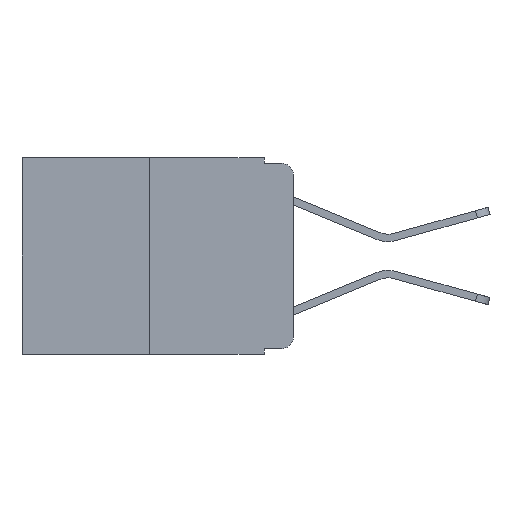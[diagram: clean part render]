
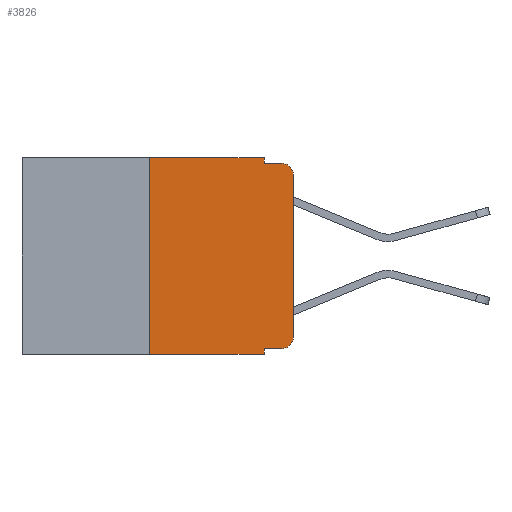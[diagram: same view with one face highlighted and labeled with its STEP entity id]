
A CAD part, left-side view. The second image highlights one B-rep face of the part: STEP entity #3826.
In plain terms, the highlighted planar face has unit normal (-1, 0, 0).
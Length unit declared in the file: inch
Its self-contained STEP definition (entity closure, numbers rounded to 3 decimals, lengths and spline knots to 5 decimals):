
#306 = CIRCLE ( 'NONE', #18237, 0.02 ) ;
#406 = VERTEX_POINT ( 'NONE', #5107 ) ;
#721 = DIRECTION ( 'NONE',  ( 0., -1., 0. ) ) ;
#767 = DIRECTION ( 'NONE',  ( 0., 0., -1. ) ) ;
#1211 = DIRECTION ( 'NONE',  ( 0., -1., 0. ) ) ;
#1782 = DIRECTION ( 'NONE',  ( 0., 0., -1. ) ) ;
#2209 = VERTEX_POINT ( 'NONE', #18327 ) ;
#2670 = VECTOR ( 'NONE', #22413, 39.37008 ) ;
#2703 = DIRECTION ( 'NONE',  ( -1., 0., 0. ) ) ;
#2939 = VECTOR ( 'NONE', #13207, 39.37008 ) ;
#3007 = CARTESIAN_POINT ( 'NONE',  ( 0., 0., 0. ) ) ;
#3672 = LINE ( 'NONE', #7604, #4236 ) ;
#3826 = ADVANCED_FACE ( 'NONE', ( #13907 ), #5703, .F. ) ;
#4138 = CARTESIAN_POINT ( 'NONE',  ( 0., 0.25, 0. ) ) ;
#4236 = VECTOR ( 'NONE', #19993, 39.37008 ) ;
#4844 = ORIENTED_EDGE ( 'NONE', *, *, #16726, .F. ) ;
#4916 = EDGE_CURVE ( 'NONE', #406, #8675, #20185, .T. ) ;
#4988 = VECTOR ( 'NONE', #721, 39.37008 ) ;
#5107 = CARTESIAN_POINT ( 'NONE',  ( 0., 0.25, -0.343 ) ) ;
#5152 = VECTOR ( 'NONE', #1782, 39.37008 ) ;
#5670 = ORIENTED_EDGE ( 'NONE', *, *, #21450, .F. ) ;
#5703 = PLANE ( 'NONE',  #8848 ) ;
#6111 = VECTOR ( 'NONE', #10324, 39.37008 ) ;
#6746 = EDGE_CURVE ( 'NONE', #7507, #6897, #306, .T. ) ;
#6845 = ORIENTED_EDGE ( 'NONE', *, *, #15632, .F. ) ;
#6897 = VERTEX_POINT ( 'NONE', #14021 ) ;
#7507 = VERTEX_POINT ( 'NONE', #19129 ) ;
#7604 = CARTESIAN_POINT ( 'NONE',  ( 0., 0.051, -0.01 ) ) ;
#7939 = EDGE_CURVE ( 'NONE', #21183, #7507, #10898, .T. ) ;
#7943 = CARTESIAN_POINT ( 'NONE',  ( 0., 0.051, -0.333 ) ) ;
#8013 = CARTESIAN_POINT ( 'NONE',  ( 0., 0.473, 0. ) ) ;
#8180 = DIRECTION ( 'NONE',  ( 0., 0., -1. ) ) ;
#8362 = LINE ( 'NONE', #9978, #13095 ) ;
#8675 = VERTEX_POINT ( 'NONE', #19466 ) ;
#8848 = AXIS2_PLACEMENT_3D ( 'NONE', #8013, #17214, #8180 ) ;
#9668 = ORIENTED_EDGE ( 'NONE', *, *, #15588, .T. ) ;
#9942 = ORIENTED_EDGE ( 'NONE', *, *, #7939, .T. ) ;
#9978 = CARTESIAN_POINT ( 'NONE',  ( 0., 0.051, 0. ) ) ;
#10151 = CARTESIAN_POINT ( 'NONE',  ( 0., 0., -0.313 ) ) ;
#10163 = VERTEX_POINT ( 'NONE', #11157 ) ;
#10324 = DIRECTION ( 'NONE',  ( 0., 0., 1. ) ) ;
#10366 = CARTESIAN_POINT ( 'NONE',  ( 0., 0.473, -0.343 ) ) ;
#10557 = LINE ( 'NONE', #10953, #5152 ) ;
#10720 = CIRCLE ( 'NONE', #17470, 0.02 ) ;
#10737 = CARTESIAN_POINT ( 'NONE',  ( 0., 0.02, -0.333 ) ) ;
#10898 = LINE ( 'NONE', #3007, #6111 ) ;
#10953 = CARTESIAN_POINT ( 'NONE',  ( 0., 0.051, 0. ) ) ;
#11157 = CARTESIAN_POINT ( 'NONE',  ( 0., 0.051, -0.01 ) ) ;
#11743 = DIRECTION ( 'NONE',  ( -1., 0., 0. ) ) ;
#11892 = CARTESIAN_POINT ( 'NONE',  ( 0., 0.25, 0. ) ) ;
#13095 = VECTOR ( 'NONE', #20552, 39.37008 ) ;
#13207 = DIRECTION ( 'NONE',  ( 0., 0., 1. ) ) ;
#13486 = CARTESIAN_POINT ( 'NONE',  ( 0., 0.051, -0.333 ) ) ;
#13560 = CARTESIAN_POINT ( 'NONE',  ( 0., 0.02, -0.03 ) ) ;
#13700 = LINE ( 'NONE', #4138, #2939 ) ;
#13907 = FACE_OUTER_BOUND ( 'NONE', #20303, .T. ) ;
#14021 = CARTESIAN_POINT ( 'NONE',  ( 0., 0.02, -0.01 ) ) ;
#14376 = EDGE_CURVE ( 'NONE', #21961, #21183, #10720, .T. ) ;
#14422 = VERTEX_POINT ( 'NONE', #11892 ) ;
#14671 = ORIENTED_EDGE ( 'NONE', *, *, #6746, .T. ) ;
#15352 = DIRECTION ( 'NONE',  ( 0., 0., -1. ) ) ;
#15588 = EDGE_CURVE ( 'NONE', #22804, #21961, #18105, .T. ) ;
#15632 = EDGE_CURVE ( 'NONE', #14422, #2209, #17564, .T. ) ;
#16633 = VECTOR ( 'NONE', #1211, 39.37008 ) ;
#16726 = EDGE_CURVE ( 'NONE', #22804, #8675, #8362, .T. ) ;
#17214 = DIRECTION ( 'NONE',  ( 1., 0., 0. ) ) ;
#17470 = AXIS2_PLACEMENT_3D ( 'NONE', #22300, #11743, #767 ) ;
#17564 = LINE ( 'NONE', #22333, #2670 ) ;
#17962 = ORIENTED_EDGE ( 'NONE', *, *, #4916, .T. ) ;
#18105 = LINE ( 'NONE', #13486, #4988 ) ;
#18237 = AXIS2_PLACEMENT_3D ( 'NONE', #13560, #2703, #15352 ) ;
#18327 = CARTESIAN_POINT ( 'NONE',  ( 0., 0.051, 0. ) ) ;
#19074 = ORIENTED_EDGE ( 'NONE', *, *, #14376, .T. ) ;
#19086 = EDGE_CURVE ( 'NONE', #406, #14422, #13700, .T. ) ;
#19129 = CARTESIAN_POINT ( 'NONE',  ( 0., 0., -0.03 ) ) ;
#19466 = CARTESIAN_POINT ( 'NONE',  ( 0., 0.051, -0.343 ) ) ;
#19993 = DIRECTION ( 'NONE',  ( 0., -1., 0. ) ) ;
#20185 = LINE ( 'NONE', #10366, #16633 ) ;
#20247 = EDGE_CURVE ( 'NONE', #2209, #10163, #10557, .T. ) ;
#20303 = EDGE_LOOP ( 'NONE', ( #9942, #14671, #5670, #20440, #6845, #21548, #17962, #4844, #9668, #19074 ) ) ;
#20440 = ORIENTED_EDGE ( 'NONE', *, *, #20247, .F. ) ;
#20552 = DIRECTION ( 'NONE',  ( 0., 0., -1. ) ) ;
#21183 = VERTEX_POINT ( 'NONE', #10151 ) ;
#21450 = EDGE_CURVE ( 'NONE', #10163, #6897, #3672, .T. ) ;
#21548 = ORIENTED_EDGE ( 'NONE', *, *, #19086, .F. ) ;
#21961 = VERTEX_POINT ( 'NONE', #10737 ) ;
#22300 = CARTESIAN_POINT ( 'NONE',  ( 0., 0.02, -0.313 ) ) ;
#22333 = CARTESIAN_POINT ( 'NONE',  ( 0., 0.473, 0. ) ) ;
#22413 = DIRECTION ( 'NONE',  ( 0., -1., 0. ) ) ;
#22804 = VERTEX_POINT ( 'NONE', #7943 ) ;
